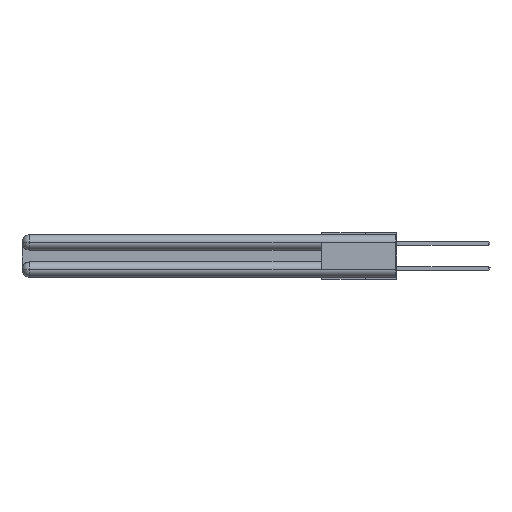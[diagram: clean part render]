
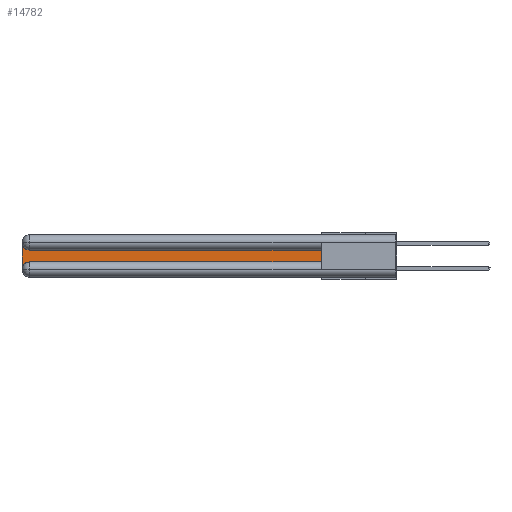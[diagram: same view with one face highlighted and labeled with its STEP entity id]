
A CAD part, left-side view. The second image highlights one B-rep face of the part: STEP entity #14782.
In plain terms, the highlighted planar face has unit normal (-1, 0, 0).
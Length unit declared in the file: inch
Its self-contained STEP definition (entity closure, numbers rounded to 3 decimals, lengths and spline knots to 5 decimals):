
#246 = VECTOR ( 'NONE', #17630, 39.37008 ) ;
#426 = CARTESIAN_POINT ( 'NONE',  ( 0.075, 3., -0.2775 ) ) ;
#668 = LINE ( 'NONE', #20939, #22230 ) ;
#1978 = EDGE_LOOP ( 'NONE', ( #30862, #23219, #16101, #33404, #17898, #33195 ) ) ;
#2057 = CARTESIAN_POINT ( 'NONE',  ( 0.075, 3., -0.0625 ) ) ;
#2285 = VERTEX_POINT ( 'NONE', #7651 ) ;
#3420 = CARTESIAN_POINT ( 'NONE',  ( 0.075, 2.94, -0.2175 ) ) ;
#4615 = AXIS2_PLACEMENT_3D ( 'NONE', #29488, #24250, #13279 ) ;
#4695 = DIRECTION ( 'NONE',  ( 0., 0., 1. ) ) ;
#4807 = DIRECTION ( 'NONE',  ( 0., -1., 0. ) ) ;
#6812 = EDGE_CURVE ( 'NONE', #2285, #26214, #12418, .T. ) ;
#6939 = DIRECTION ( 'NONE',  ( 1., 0., 0. ) ) ;
#7651 = CARTESIAN_POINT ( 'NONE',  ( 0.075, 2.94, -0.1225 ) ) ;
#8871 = FACE_OUTER_BOUND ( 'NONE', #1978, .T. ) ;
#9124 = DIRECTION ( 'NONE',  ( 0., 0., -1. ) ) ;
#9629 = DIRECTION ( 'NONE',  ( 0., 0., -1. ) ) ;
#11831 = CARTESIAN_POINT ( 'NONE',  ( 0.075, 3., -0.2175 ) ) ;
#11972 = CARTESIAN_POINT ( 'NONE',  ( 0.075, 0.6, -0.1225 ) ) ;
#12418 = CIRCLE ( 'NONE', #31854, 0.06 ) ;
#13279 = DIRECTION ( 'NONE',  ( 0., 0., -1. ) ) ;
#14782 = ADVANCED_FACE ( 'NONE', ( #8871 ), #30956, .F. ) ;
#16101 = ORIENTED_EDGE ( 'NONE', *, *, #25967, .T. ) ;
#16927 = VERTEX_POINT ( 'NONE', #3420 ) ;
#17587 = LINE ( 'NONE', #11972, #246 ) ;
#17630 = DIRECTION ( 'NONE',  ( 0., 1., 0. ) ) ;
#17898 = ORIENTED_EDGE ( 'NONE', *, *, #23249, .T. ) ;
#19856 = CARTESIAN_POINT ( 'NONE',  ( 0.075, 2.94, -0.0625 ) ) ;
#20279 = EDGE_CURVE ( 'NONE', #23542, #30066, #23707, .T. ) ;
#20460 = CARTESIAN_POINT ( 'NONE',  ( 0.075, 3., -0.1225 ) ) ;
#20939 = CARTESIAN_POINT ( 'NONE',  ( 0.075, 0.6, -0.2175 ) ) ;
#21970 = AXIS2_PLACEMENT_3D ( 'NONE', #20460, #6939, #9629 ) ;
#22230 = VECTOR ( 'NONE', #4807, 39.37008 ) ;
#22348 = VERTEX_POINT ( 'NONE', #426 ) ;
#22360 = DIRECTION ( 'NONE',  ( 1., 0., 0. ) ) ;
#23219 = ORIENTED_EDGE ( 'NONE', *, *, #6812, .T. ) ;
#23249 = EDGE_CURVE ( 'NONE', #16927, #23542, #668, .T. ) ;
#23542 = VERTEX_POINT ( 'NONE', #28918 ) ;
#23707 = LINE ( 'NONE', #29410, #31817 ) ;
#24096 = CARTESIAN_POINT ( 'NONE',  ( 0.075, 0.6, -0.1225 ) ) ;
#24250 = DIRECTION ( 'NONE',  ( 1., 0., 0. ) ) ;
#24486 = EDGE_CURVE ( 'NONE', #22348, #16927, #30855, .T. ) ;
#25662 = LINE ( 'NONE', #11831, #32082 ) ;
#25967 = EDGE_CURVE ( 'NONE', #26214, #22348, #25662, .T. ) ;
#26214 = VERTEX_POINT ( 'NONE', #2057 ) ;
#26547 = EDGE_CURVE ( 'NONE', #30066, #2285, #17587, .T. ) ;
#27912 = DIRECTION ( 'NONE',  ( 0., 0., -1. ) ) ;
#28918 = CARTESIAN_POINT ( 'NONE',  ( 0.075, 0.6, -0.2175 ) ) ;
#29410 = CARTESIAN_POINT ( 'NONE',  ( 0.075, 0.6, -0.2175 ) ) ;
#29488 = CARTESIAN_POINT ( 'NONE',  ( 0.075, 2.94, -0.2775 ) ) ;
#30066 = VERTEX_POINT ( 'NONE', #24096 ) ;
#30855 = CIRCLE ( 'NONE', #4615, 0.06 ) ;
#30862 = ORIENTED_EDGE ( 'NONE', *, *, #26547, .T. ) ;
#30956 = PLANE ( 'NONE',  #21970 ) ;
#31817 = VECTOR ( 'NONE', #4695, 39.37008 ) ;
#31854 = AXIS2_PLACEMENT_3D ( 'NONE', #19856, #22360, #9124 ) ;
#32082 = VECTOR ( 'NONE', #27912, 39.37008 ) ;
#33195 = ORIENTED_EDGE ( 'NONE', *, *, #20279, .T. ) ;
#33404 = ORIENTED_EDGE ( 'NONE', *, *, #24486, .T. ) ;
